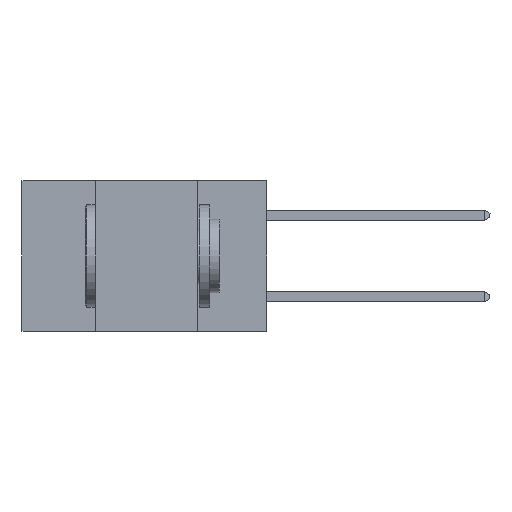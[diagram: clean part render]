
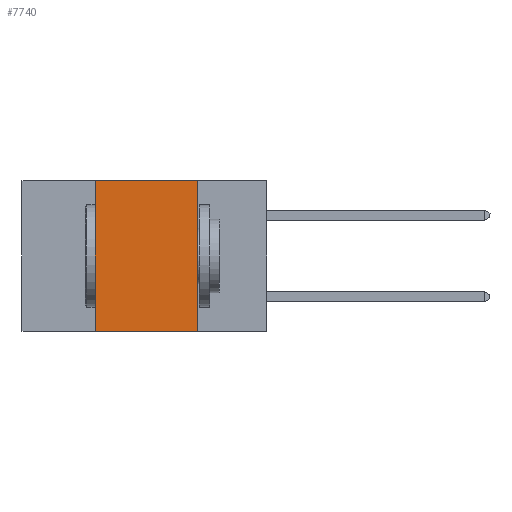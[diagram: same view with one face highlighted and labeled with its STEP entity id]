
A CAD part, left-side view. The second image highlights one B-rep face of the part: STEP entity #7740.
In plain terms, the highlighted planar face has unit normal (-1, 0, 0).
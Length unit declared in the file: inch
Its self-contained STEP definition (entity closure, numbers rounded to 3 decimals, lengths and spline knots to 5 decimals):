
#1292 = EDGE_CURVE ( 'NONE', #10322, #4511, #2965, .T. ) ;
#1293 = DIRECTION ( 'NONE',  ( 0., 0., -1. ) ) ;
#1670 = CARTESIAN_POINT ( 'NONE',  ( 0., 0.6, -0.37 ) ) ;
#2145 = VECTOR ( 'NONE', #1293, 39.37008 ) ;
#2347 = CARTESIAN_POINT ( 'NONE',  ( 0., 0.17, 0. ) ) ;
#2615 = DIRECTION ( 'NONE',  ( 0., -1., 0. ) ) ;
#2965 = LINE ( 'NONE', #4122, #9153 ) ;
#2982 = VERTEX_POINT ( 'NONE', #7263 ) ;
#3241 = EDGE_LOOP ( 'NONE', ( #6886, #6899, #6920, #6977 ) ) ;
#3339 = CARTESIAN_POINT ( 'NONE',  ( 0., 0.42, 0. ) ) ;
#3885 = CARTESIAN_POINT ( 'NONE',  ( 0., 0.6, 0. ) ) ;
#4122 = CARTESIAN_POINT ( 'NONE',  ( 0., 0.6, 0. ) ) ;
#4233 = VERTEX_POINT ( 'NONE', #8635 ) ;
#4366 = VECTOR ( 'NONE', #2615, 39.37008 ) ;
#4511 = VERTEX_POINT ( 'NONE', #2347 ) ;
#5324 = DIRECTION ( 'NONE',  ( 0., 0., 1. ) ) ;
#5678 = DIRECTION ( 'NONE',  ( 0., 0., -1. ) ) ;
#5808 = CARTESIAN_POINT ( 'NONE',  ( 0., 0.17, 0. ) ) ;
#6364 = EDGE_CURVE ( 'NONE', #4511, #2982, #10741, .T. ) ;
#6689 = LINE ( 'NONE', #10890, #8806 ) ;
#6761 = EDGE_CURVE ( 'NONE', #4233, #2982, #10850, .T. ) ;
#6777 = EDGE_CURVE ( 'NONE', #4233, #10322, #6689, .T. ) ;
#6886 = ORIENTED_EDGE ( 'NONE', *, *, #6364, .F. ) ;
#6899 = ORIENTED_EDGE ( 'NONE', *, *, #1292, .F. ) ;
#6920 = ORIENTED_EDGE ( 'NONE', *, *, #6777, .F. ) ;
#6977 = ORIENTED_EDGE ( 'NONE', *, *, #6761, .T. ) ;
#7127 = DIRECTION ( 'NONE',  ( 0., -1., 0. ) ) ;
#7263 = CARTESIAN_POINT ( 'NONE',  ( 0., 0.17, -0.37 ) ) ;
#7740 = ADVANCED_FACE ( 'NONE', ( #8424 ), #8890, .F. ) ;
#8424 = FACE_OUTER_BOUND ( 'NONE', #3241, .T. ) ;
#8635 = CARTESIAN_POINT ( 'NONE',  ( 0., 0.42, -0.37 ) ) ;
#8806 = VECTOR ( 'NONE', #5324, 39.37008 ) ;
#8890 = PLANE ( 'NONE',  #9725 ) ;
#9153 = VECTOR ( 'NONE', #7127, 39.37008 ) ;
#9725 = AXIS2_PLACEMENT_3D ( 'NONE', #3885, #10460, #5678 ) ;
#10322 = VERTEX_POINT ( 'NONE', #3339 ) ;
#10460 = DIRECTION ( 'NONE',  ( 1., 0., 0. ) ) ;
#10741 = LINE ( 'NONE', #5808, #2145 ) ;
#10850 = LINE ( 'NONE', #1670, #4366 ) ;
#10890 = CARTESIAN_POINT ( 'NONE',  ( 0., 0.42, 0. ) ) ;
